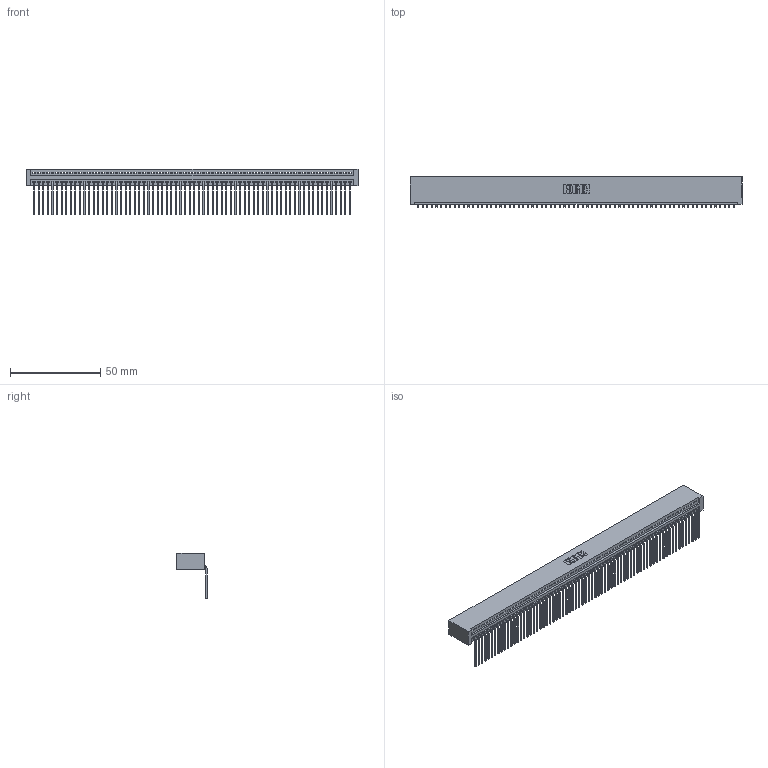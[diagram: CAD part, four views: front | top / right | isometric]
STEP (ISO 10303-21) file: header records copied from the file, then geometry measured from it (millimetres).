
FILE_DESCRIPTION (( 'STEP AP203' ), '1' );
FILE_NAME ('395-070-559-101.STEP', '2019-10-26T02:23:17', ( '' ), ( '' ), 'SwSTEP 2.0', 'SolidWorks 2016', '' );
FILE_SCHEMA (( 'CONFIG_CONTROL_DESIGN' ));
Length unit declared in the file: inch
Products named in the file (3): 395-070-559-101; 345 Part_No Mounting Lugs; 345-292-001_558 559 Tail - 1
Assembly tree (71 placements, depth 2):
  395-070-559-101
    345 Part_No Mounting Lugs
    345-292-001_558 559 Tail - 1  x70
Bounding box: 184.4 x 16.75 x 25.53 mm (x, y, z)
Volume: 18561.8 mm3; surface area: 26608.1 mm2
Topology: 71 solids, 71 shells, 4318 faces, 13057 edges, 8610 vertices
Faces by surface type: plane 3016, cylinder 1302
Entity records: 48721 total; most frequent: ORIENTED_EDGE 8450, CARTESIAN_POINT 8446, DIRECTION 7329, EDGE_CURVE 4225, VECTOR 3821, LINE 3821, VERTEX_POINT 2814, AXIS2_PLACEMENT_3D 1754
